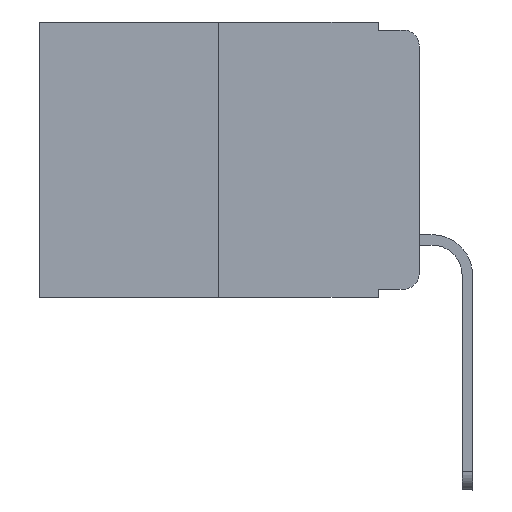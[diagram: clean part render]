
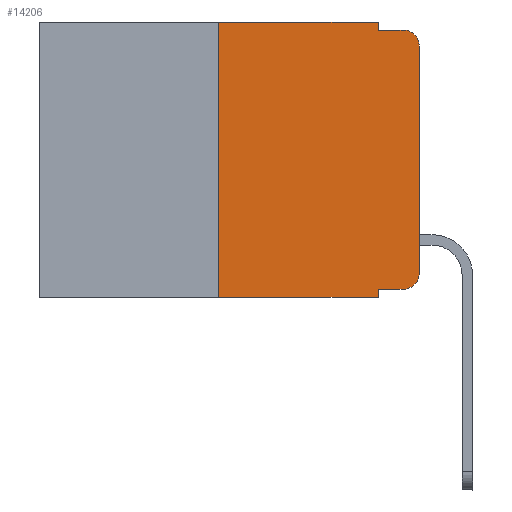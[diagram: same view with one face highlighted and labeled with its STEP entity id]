
A CAD part, left-side view. The second image highlights one B-rep face of the part: STEP entity #14206.
In plain terms, the highlighted planar face has unit normal (-1, 0, 0).
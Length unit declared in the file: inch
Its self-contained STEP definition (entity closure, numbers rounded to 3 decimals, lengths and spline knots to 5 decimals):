
#88 = DIRECTION ( 'NONE',  ( -1., 0., 0. ) ) ;
#278 = ORIENTED_EDGE ( 'NONE', *, *, #11816, .T. ) ;
#350 = VERTEX_POINT ( 'NONE', #14587 ) ;
#406 = CARTESIAN_POINT ( 'NONE',  ( 0., 0., -0.03 ) ) ;
#572 = DIRECTION ( 'NONE',  ( 1., 0., 0. ) ) ;
#633 = LINE ( 'NONE', #10005, #5850 ) ;
#865 = DIRECTION ( 'NONE',  ( 0., 0., 1. ) ) ;
#904 = CARTESIAN_POINT ( 'NONE',  ( 0., 0.473, -0.343 ) ) ;
#1033 = CARTESIAN_POINT ( 'NONE',  ( 0., 0.051, -0.01 ) ) ;
#1442 = EDGE_CURVE ( 'NONE', #14508, #350, #3625, .T. ) ;
#1486 = CIRCLE ( 'NONE', #5494, 0.02 ) ;
#1694 = EDGE_LOOP ( 'NONE', ( #278, #11307, #11073, #14022, #8560, #7207, #12187, #13707, #2631, #8464 ) ) ;
#1705 = VECTOR ( 'NONE', #5965, 39.37008 ) ;
#1957 = CARTESIAN_POINT ( 'NONE',  ( 0., 0.25, -0.343 ) ) ;
#1974 = VECTOR ( 'NONE', #865, 39.37008 ) ;
#2441 = LINE ( 'NONE', #6212, #4035 ) ;
#2631 = ORIENTED_EDGE ( 'NONE', *, *, #11613, .T. ) ;
#2868 = CARTESIAN_POINT ( 'NONE',  ( 0., 0.051, -0.01 ) ) ;
#2922 = FACE_OUTER_BOUND ( 'NONE', #1694, .T. ) ;
#3098 = VECTOR ( 'NONE', #12989, 39.37008 ) ;
#3504 = EDGE_CURVE ( 'NONE', #6031, #12512, #11625, .T. ) ;
#3517 = DIRECTION ( 'NONE',  ( 0., 0., -1. ) ) ;
#3620 = CARTESIAN_POINT ( 'NONE',  ( 0., 0.25, 0. ) ) ;
#3625 = LINE ( 'NONE', #8198, #3098 ) ;
#3719 = EDGE_CURVE ( 'NONE', #14242, #8905, #8936, .T. ) ;
#4035 = VECTOR ( 'NONE', #7241, 39.37008 ) ;
#4175 = VERTEX_POINT ( 'NONE', #406 ) ;
#4648 = CARTESIAN_POINT ( 'NONE',  ( 0., 0., 0. ) ) ;
#5253 = VERTEX_POINT ( 'NONE', #5333 ) ;
#5282 = LINE ( 'NONE', #12604, #10758 ) ;
#5333 = CARTESIAN_POINT ( 'NONE',  ( 0., 0.02, -0.333 ) ) ;
#5428 = CARTESIAN_POINT ( 'NONE',  ( 0., 0.25, 0. ) ) ;
#5494 = AXIS2_PLACEMENT_3D ( 'NONE', #14725, #88, #7486 ) ;
#5526 = PLANE ( 'NONE',  #14358 ) ;
#5850 = VECTOR ( 'NONE', #12600, 39.37008 ) ;
#5965 = DIRECTION ( 'NONE',  ( 0., 0., 1. ) ) ;
#6031 = VERTEX_POINT ( 'NONE', #1957 ) ;
#6212 = CARTESIAN_POINT ( 'NONE',  ( 0., 0.051, 0. ) ) ;
#6335 = VECTOR ( 'NONE', #9492, 39.37008 ) ;
#7207 = ORIENTED_EDGE ( 'NONE', *, *, #9369, .F. ) ;
#7241 = DIRECTION ( 'NONE',  ( 0., 0., -1. ) ) ;
#7486 = DIRECTION ( 'NONE',  ( 0., 0., -1. ) ) ;
#8048 = DIRECTION ( 'NONE',  ( 0., 0., -1. ) ) ;
#8198 = CARTESIAN_POINT ( 'NONE',  ( 0., 0.473, 0. ) ) ;
#8464 = ORIENTED_EDGE ( 'NONE', *, *, #10341, .T. ) ;
#8560 = ORIENTED_EDGE ( 'NONE', *, *, #1442, .F. ) ;
#8905 = VERTEX_POINT ( 'NONE', #13217 ) ;
#8936 = LINE ( 'NONE', #2868, #11287 ) ;
#9062 = EDGE_CURVE ( 'NONE', #11229, #12512, #633, .T. ) ;
#9369 = EDGE_CURVE ( 'NONE', #6031, #14508, #10704, .T. ) ;
#9492 = DIRECTION ( 'NONE',  ( 0., -1., 0. ) ) ;
#9528 = LINE ( 'NONE', #4648, #1974 ) ;
#10005 = CARTESIAN_POINT ( 'NONE',  ( 0., 0.051, 0. ) ) ;
#10341 = EDGE_CURVE ( 'NONE', #5253, #12815, #1486, .T. ) ;
#10370 = CIRCLE ( 'NONE', #13149, 0.02 ) ;
#10409 = CARTESIAN_POINT ( 'NONE',  ( 0., 0.473, 0. ) ) ;
#10682 = CARTESIAN_POINT ( 'NONE',  ( 0., 0.02, -0.03 ) ) ;
#10704 = LINE ( 'NONE', #3620, #1705 ) ;
#10758 = VECTOR ( 'NONE', #12449, 39.37008 ) ;
#11073 = ORIENTED_EDGE ( 'NONE', *, *, #3719, .F. ) ;
#11229 = VERTEX_POINT ( 'NONE', #13827 ) ;
#11287 = VECTOR ( 'NONE', #12400, 39.37008 ) ;
#11307 = ORIENTED_EDGE ( 'NONE', *, *, #15190, .T. ) ;
#11613 = EDGE_CURVE ( 'NONE', #11229, #5253, #5282, .T. ) ;
#11625 = LINE ( 'NONE', #904, #6335 ) ;
#11816 = EDGE_CURVE ( 'NONE', #12815, #4175, #9528, .T. ) ;
#12187 = ORIENTED_EDGE ( 'NONE', *, *, #3504, .T. ) ;
#12400 = DIRECTION ( 'NONE',  ( 0., -1., 0. ) ) ;
#12449 = DIRECTION ( 'NONE',  ( 0., -1., 0. ) ) ;
#12512 = VERTEX_POINT ( 'NONE', #12645 ) ;
#12600 = DIRECTION ( 'NONE',  ( 0., 0., -1. ) ) ;
#12604 = CARTESIAN_POINT ( 'NONE',  ( 0., 0.051, -0.333 ) ) ;
#12645 = CARTESIAN_POINT ( 'NONE',  ( 0., 0.051, -0.343 ) ) ;
#12815 = VERTEX_POINT ( 'NONE', #14513 ) ;
#12989 = DIRECTION ( 'NONE',  ( 0., -1., 0. ) ) ;
#13149 = AXIS2_PLACEMENT_3D ( 'NONE', #10682, #15477, #3517 ) ;
#13202 = EDGE_CURVE ( 'NONE', #350, #14242, #2441, .T. ) ;
#13217 = CARTESIAN_POINT ( 'NONE',  ( 0., 0.02, -0.01 ) ) ;
#13707 = ORIENTED_EDGE ( 'NONE', *, *, #9062, .F. ) ;
#13827 = CARTESIAN_POINT ( 'NONE',  ( 0., 0.051, -0.333 ) ) ;
#14022 = ORIENTED_EDGE ( 'NONE', *, *, #13202, .F. ) ;
#14206 = ADVANCED_FACE ( 'NONE', ( #2922 ), #5526, .F. ) ;
#14242 = VERTEX_POINT ( 'NONE', #1033 ) ;
#14358 = AXIS2_PLACEMENT_3D ( 'NONE', #10409, #572, #8048 ) ;
#14508 = VERTEX_POINT ( 'NONE', #5428 ) ;
#14513 = CARTESIAN_POINT ( 'NONE',  ( 0., 0., -0.313 ) ) ;
#14587 = CARTESIAN_POINT ( 'NONE',  ( 0., 0.051, 0. ) ) ;
#14725 = CARTESIAN_POINT ( 'NONE',  ( 0., 0.02, -0.313 ) ) ;
#15190 = EDGE_CURVE ( 'NONE', #4175, #8905, #10370, .T. ) ;
#15477 = DIRECTION ( 'NONE',  ( -1., 0., 0. ) ) ;
